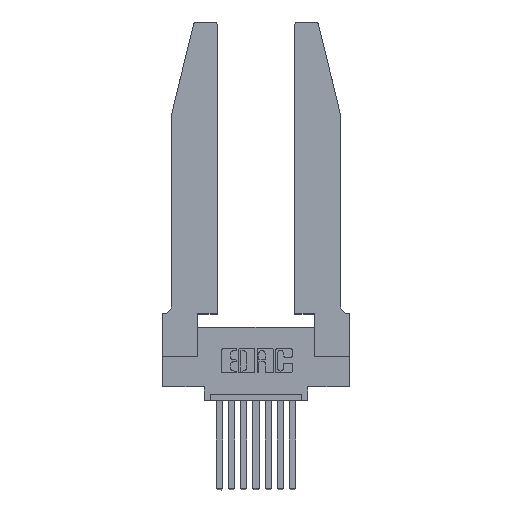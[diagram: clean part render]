
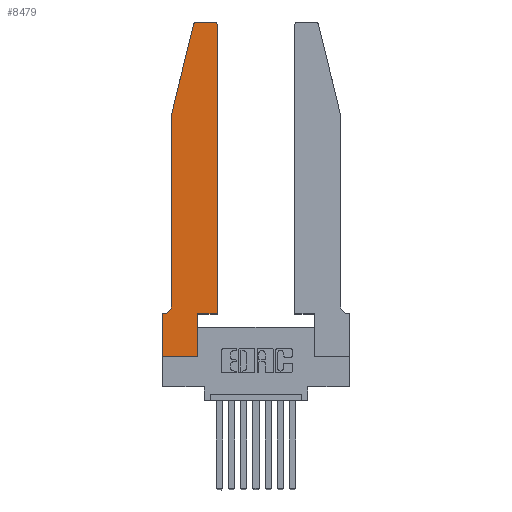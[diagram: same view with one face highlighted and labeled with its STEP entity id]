
A CAD part, top view. The second image highlights one B-rep face of the part: STEP entity #8479.
In plain terms, the highlighted planar face has unit normal (0, 0, 1).
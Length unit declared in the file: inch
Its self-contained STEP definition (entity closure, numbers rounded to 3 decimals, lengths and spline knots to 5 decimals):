
#108 = CARTESIAN_POINT ( 'NONE',  ( 0.2865, 0., 0.37 ) ) ;
#283 = DIRECTION ( 'NONE',  ( 1., 0., 0. ) ) ;
#952 = VERTEX_POINT ( 'NONE', #1116 ) ;
#956 = LINE ( 'NONE', #6055, #7002 ) ;
#1089 = CARTESIAN_POINT ( 'NONE',  ( 0.284, 2.72, 0.37 ) ) ;
#1116 = CARTESIAN_POINT ( 'NONE',  ( 0.2865, 0.35, 0.37 ) ) ;
#1317 = DIRECTION ( 'NONE',  ( -0.239, -0.971, 0. ) ) ;
#1320 = VERTEX_POINT ( 'NONE', #7008 ) ;
#1410 = CARTESIAN_POINT ( 'NONE',  ( 0.0755, 2., 0.37 ) ) ;
#1430 = CARTESIAN_POINT ( 'NONE',  ( 0.4205, 2.75, 0.37 ) ) ;
#1610 = VECTOR ( 'NONE', #3918, 39.37008 ) ;
#1782 = EDGE_CURVE ( 'NONE', #8914, #7215, #2795, .T. ) ;
#1853 = ORIENTED_EDGE ( 'NONE', *, *, #3851, .T. ) ;
#2090 = LINE ( 'NONE', #14077, #12572 ) ;
#2201 = CIRCLE ( 'NONE', #6186, 0.07 ) ;
#2321 = VERTEX_POINT ( 'NONE', #8229 ) ;
#2331 = EDGE_CURVE ( 'NONE', #13167, #2334, #4561, .T. ) ;
#2334 = VERTEX_POINT ( 'NONE', #1430 ) ;
#2642 = LINE ( 'NONE', #3132, #9598 ) ;
#2720 = DIRECTION ( 'NONE',  ( -1., 0., 0. ) ) ;
#2795 = CIRCLE ( 'NONE', #4645, 0.03 ) ;
#2924 = ORIENTED_EDGE ( 'NONE', *, *, #4962, .T. ) ;
#2928 = DIRECTION ( 'NONE',  ( -1., 0., 0. ) ) ;
#2984 = DIRECTION ( 'NONE',  ( 0., -1., 0. ) ) ;
#3029 = ORIENTED_EDGE ( 'NONE', *, *, #5931, .T. ) ;
#3132 = CARTESIAN_POINT ( 'NONE',  ( 0., 0., 0.37 ) ) ;
#3492 = ORIENTED_EDGE ( 'NONE', *, *, #10489, .T. ) ;
#3582 = ORIENTED_EDGE ( 'NONE', *, *, #2331, .T. ) ;
#3851 = EDGE_CURVE ( 'NONE', #8628, #952, #6672, .T. ) ;
#3918 = DIRECTION ( 'NONE',  ( 0., -1., 0. ) ) ;
#4015 = FACE_OUTER_BOUND ( 'NONE', #5649, .T. ) ;
#4217 = VECTOR ( 'NONE', #9749, 39.37008 ) ;
#4293 = CARTESIAN_POINT ( 'NONE',  ( 0.284, 2.75, 0.37 ) ) ;
#4561 = CIRCLE ( 'NONE', #5319, 0.03 ) ;
#4645 = AXIS2_PLACEMENT_3D ( 'NONE', #1089, #6761, #12263 ) ;
#4667 = ORIENTED_EDGE ( 'NONE', *, *, #7442, .T. ) ;
#4962 = EDGE_CURVE ( 'NONE', #6545, #6910, #2201, .T. ) ;
#5319 = AXIS2_PLACEMENT_3D ( 'NONE', #7145, #7196, #283 ) ;
#5507 = ORIENTED_EDGE ( 'NONE', *, *, #6111, .T. ) ;
#5533 = PLANE ( 'NONE',  #10536 ) ;
#5649 = EDGE_LOOP ( 'NONE', ( #5507, #12877, #8489, #4667, #2924, #3492, #3029, #6845, #1853, #11009, #13488, #3582 ) ) ;
#5657 = DIRECTION ( 'NONE',  ( 0., 1., 0. ) ) ;
#5678 = CARTESIAN_POINT ( 'NONE',  ( 0.25487, 2.72718, 0.37 ) ) ;
#5889 = LINE ( 'NONE', #11315, #9275 ) ;
#5931 = EDGE_CURVE ( 'NONE', #2321, #10461, #9464, .T. ) ;
#6055 = CARTESIAN_POINT ( 'NONE',  ( 0.0755, 0.35, 0.37 ) ) ;
#6111 = EDGE_CURVE ( 'NONE', #2334, #8914, #5889, .T. ) ;
#6186 = AXIS2_PLACEMENT_3D ( 'NONE', #9699, #10927, #2928 ) ;
#6244 = CARTESIAN_POINT ( 'NONE',  ( 0., 0., 0.37 ) ) ;
#6297 = VECTOR ( 'NONE', #5657, 39.37008 ) ;
#6390 = CARTESIAN_POINT ( 'NONE',  ( 0.0755, 2., 0.37 ) ) ;
#6545 = VERTEX_POINT ( 'NONE', #10040 ) ;
#6672 = LINE ( 'NONE', #11317, #6297 ) ;
#6761 = DIRECTION ( 'NONE',  ( 0., 0., 1. ) ) ;
#6845 = ORIENTED_EDGE ( 'NONE', *, *, #13455, .T. ) ;
#6910 = VERTEX_POINT ( 'NONE', #10714 ) ;
#7002 = VECTOR ( 'NONE', #2720, 39.37008 ) ;
#7008 = CARTESIAN_POINT ( 'NONE',  ( 0.4505, 0.35, 0.37 ) ) ;
#7062 = LINE ( 'NONE', #8772, #4217 ) ;
#7145 = CARTESIAN_POINT ( 'NONE',  ( 0.4205, 2.72, 0.37 ) ) ;
#7196 = DIRECTION ( 'NONE',  ( 0., 0., 1. ) ) ;
#7215 = VERTEX_POINT ( 'NONE', #5678 ) ;
#7295 = CARTESIAN_POINT ( 'NONE',  ( 0., 0., 0.37 ) ) ;
#7442 = EDGE_CURVE ( 'NONE', #12223, #6545, #2090, .T. ) ;
#7765 = DIRECTION ( 'NONE',  ( 1., 0., 0. ) ) ;
#7789 = VECTOR ( 'NONE', #1317, 39.37008 ) ;
#7894 = EDGE_CURVE ( 'NONE', #952, #1320, #7062, .T. ) ;
#8136 = LINE ( 'NONE', #1410, #7789 ) ;
#8229 = CARTESIAN_POINT ( 'NONE',  ( 0., 0.35, 0.37 ) ) ;
#8479 = ADVANCED_FACE ( 'NONE', ( #4015 ), #5533, .T. ) ;
#8489 = ORIENTED_EDGE ( 'NONE', *, *, #14046, .T. ) ;
#8628 = VERTEX_POINT ( 'NONE', #108 ) ;
#8694 = DIRECTION ( 'NONE',  ( 0., 1., 0. ) ) ;
#8772 = CARTESIAN_POINT ( 'NONE',  ( 0.4505, 0.35, 0.37 ) ) ;
#8904 = CARTESIAN_POINT ( 'NONE',  ( 0., 0.35, 0.37 ) ) ;
#8914 = VERTEX_POINT ( 'NONE', #4293 ) ;
#9275 = VECTOR ( 'NONE', #13436, 39.37008 ) ;
#9464 = LINE ( 'NONE', #6244, #1610 ) ;
#9564 = CARTESIAN_POINT ( 'NONE',  ( 0.4505, 2.72, 0.37 ) ) ;
#9598 = VECTOR ( 'NONE', #10054, 39.37008 ) ;
#9699 = CARTESIAN_POINT ( 'NONE',  ( 0.0055, 0.42, 0.37 ) ) ;
#9749 = DIRECTION ( 'NONE',  ( 1., 0., 0. ) ) ;
#9753 = EDGE_CURVE ( 'NONE', #1320, #13167, #13042, .T. ) ;
#10040 = CARTESIAN_POINT ( 'NONE',  ( 0.0755, 0.42, 0.37 ) ) ;
#10054 = DIRECTION ( 'NONE',  ( 1., 0., 0. ) ) ;
#10070 = DIRECTION ( 'NONE',  ( 0., 0., 1. ) ) ;
#10461 = VERTEX_POINT ( 'NONE', #7295 ) ;
#10489 = EDGE_CURVE ( 'NONE', #6910, #2321, #956, .T. ) ;
#10536 = AXIS2_PLACEMENT_3D ( 'NONE', #8904, #10070, #7765 ) ;
#10714 = CARTESIAN_POINT ( 'NONE',  ( 0.0055, 0.35, 0.37 ) ) ;
#10927 = DIRECTION ( 'NONE',  ( 0., 0., -1. ) ) ;
#11009 = ORIENTED_EDGE ( 'NONE', *, *, #7894, .T. ) ;
#11111 = VECTOR ( 'NONE', #8694, 39.37008 ) ;
#11315 = CARTESIAN_POINT ( 'NONE',  ( 0.2605, 2.75, 0.37 ) ) ;
#11317 = CARTESIAN_POINT ( 'NONE',  ( 0.2865, 0.35, 0.37 ) ) ;
#12030 = CARTESIAN_POINT ( 'NONE',  ( 0.4505, 0.35, 0.37 ) ) ;
#12223 = VERTEX_POINT ( 'NONE', #6390 ) ;
#12263 = DIRECTION ( 'NONE',  ( 1., 0., 0. ) ) ;
#12572 = VECTOR ( 'NONE', #2984, 39.37008 ) ;
#12877 = ORIENTED_EDGE ( 'NONE', *, *, #1782, .T. ) ;
#13042 = LINE ( 'NONE', #12030, #11111 ) ;
#13167 = VERTEX_POINT ( 'NONE', #9564 ) ;
#13436 = DIRECTION ( 'NONE',  ( -1., 0., 0. ) ) ;
#13455 = EDGE_CURVE ( 'NONE', #10461, #8628, #2642, .T. ) ;
#13488 = ORIENTED_EDGE ( 'NONE', *, *, #9753, .T. ) ;
#14046 = EDGE_CURVE ( 'NONE', #7215, #12223, #8136, .T. ) ;
#14077 = CARTESIAN_POINT ( 'NONE',  ( 0.0755, 2., 0.37 ) ) ;
